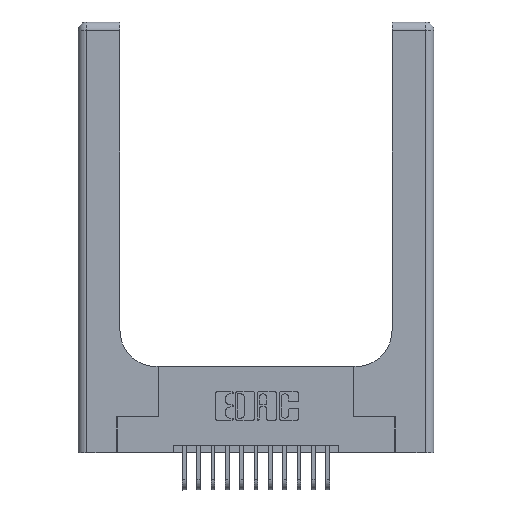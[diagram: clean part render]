
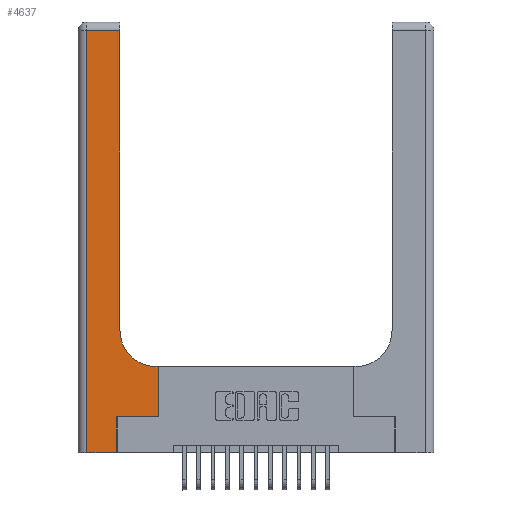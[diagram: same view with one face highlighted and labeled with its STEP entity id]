
A CAD part, top view. The second image highlights one B-rep face of the part: STEP entity #4637.
In plain terms, the highlighted planar face has unit normal (0, 0, 1).
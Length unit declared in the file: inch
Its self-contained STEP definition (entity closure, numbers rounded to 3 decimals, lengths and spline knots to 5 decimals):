
#248 = EDGE_CURVE ( 'NONE', #2853, #952, #790, .T. ) ;
#262 = LINE ( 'NONE', #1208, #7528 ) ;
#790 = LINE ( 'NONE', #9815, #4466 ) ;
#952 = VERTEX_POINT ( 'NONE', #16871 ) ;
#1208 = CARTESIAN_POINT ( 'NONE',  ( 0.269, 0.25, 0.37 ) ) ;
#1217 = ORIENTED_EDGE ( 'NONE', *, *, #9031, .T. ) ;
#1301 = CARTESIAN_POINT ( 'NONE',  ( 0.2915, 2.94, 0.37 ) ) ;
#1729 = ORIENTED_EDGE ( 'NONE', *, *, #12691, .T. ) ;
#1808 = VECTOR ( 'NONE', #4950, 39.37008 ) ;
#2254 = EDGE_CURVE ( 'NONE', #8453, #15381, #5851, .T. ) ;
#2398 = DIRECTION ( 'NONE',  ( 0., 1., 0. ) ) ;
#2740 = CARTESIAN_POINT ( 'NONE',  ( 0.5585, 0.6, 0.37 ) ) ;
#2793 = DIRECTION ( 'NONE',  ( -1., 0., 0. ) ) ;
#2853 = VERTEX_POINT ( 'NONE', #17217 ) ;
#3018 = DIRECTION ( 'NONE',  ( 0., 1., 0. ) ) ;
#3750 = VERTEX_POINT ( 'NONE', #16655 ) ;
#4372 = PLANE ( 'NONE',  #6452 ) ;
#4466 = VECTOR ( 'NONE', #14268, 39.37008 ) ;
#4471 = CARTESIAN_POINT ( 'NONE',  ( 0.2915, 3., 0.37 ) ) ;
#4545 = CARTESIAN_POINT ( 'NONE',  ( 0.5585, 0.25, 0.37 ) ) ;
#4637 = ADVANCED_FACE ( 'NONE', ( #17315 ), #4372, .F. ) ;
#4950 = DIRECTION ( 'NONE',  ( -1., 0., 0. ) ) ;
#4987 = EDGE_CURVE ( 'NONE', #15241, #11306, #12165, .T. ) ;
#4993 = VECTOR ( 'NONE', #3018, 39.37008 ) ;
#5088 = EDGE_CURVE ( 'NONE', #9762, #8453, #14529, .T. ) ;
#5576 = DIRECTION ( 'NONE',  ( 0., 0., -1. ) ) ;
#5727 = DIRECTION ( 'NONE',  ( -1., 0., 0. ) ) ;
#5851 = LINE ( 'NONE', #15827, #1808 ) ;
#6071 = DIRECTION ( 'NONE',  ( 0., -1., 0. ) ) ;
#6157 = LINE ( 'NONE', #14285, #17087 ) ;
#6452 = AXIS2_PLACEMENT_3D ( 'NONE', #8402, #13926, #5727 ) ;
#7070 = CARTESIAN_POINT ( 'NONE',  ( 0.06, 2.94, 0.37 ) ) ;
#7467 = VECTOR ( 'NONE', #2398, 39.37008 ) ;
#7528 = VECTOR ( 'NONE', #8007, 39.37008 ) ;
#8007 = DIRECTION ( 'NONE',  ( 1., 0., 0. ) ) ;
#8081 = VECTOR ( 'NONE', #14018, 39.37008 ) ;
#8162 = LINE ( 'NONE', #11180, #4993 ) ;
#8402 = CARTESIAN_POINT ( 'NONE',  ( 0., 3., 0.37 ) ) ;
#8453 = VERTEX_POINT ( 'NONE', #1301 ) ;
#8523 = VECTOR ( 'NONE', #2793, 39.37008 ) ;
#9031 = EDGE_CURVE ( 'NONE', #3750, #15424, #262, .T. ) ;
#9245 = EDGE_CURVE ( 'NONE', #15424, #15241, #8162, .T. ) ;
#9762 = VERTEX_POINT ( 'NONE', #12242 ) ;
#9815 = CARTESIAN_POINT ( 'NONE',  ( 0., 0., 0.37 ) ) ;
#10178 = EDGE_LOOP ( 'NONE', ( #13649, #10847, #17282, #11571, #13749, #1217, #10959, #10189, #1729 ) ) ;
#10189 = ORIENTED_EDGE ( 'NONE', *, *, #4987, .T. ) ;
#10813 = CARTESIAN_POINT ( 'NONE',  ( 0.5415, 0.6, 0.37 ) ) ;
#10847 = ORIENTED_EDGE ( 'NONE', *, *, #2254, .T. ) ;
#10958 = CARTESIAN_POINT ( 'NONE',  ( 0.2915, 0.6, 0.37 ) ) ;
#10959 = ORIENTED_EDGE ( 'NONE', *, *, #9245, .T. ) ;
#11180 = CARTESIAN_POINT ( 'NONE',  ( 0.5585, 0.25, 0.37 ) ) ;
#11306 = VERTEX_POINT ( 'NONE', #10813 ) ;
#11567 = CIRCLE ( 'NONE', #12018, 0.25 ) ;
#11571 = ORIENTED_EDGE ( 'NONE', *, *, #248, .T. ) ;
#12018 = AXIS2_PLACEMENT_3D ( 'NONE', #13751, #5576, #15139 ) ;
#12165 = LINE ( 'NONE', #10958, #8523 ) ;
#12242 = CARTESIAN_POINT ( 'NONE',  ( 0.2915, 0.85, 0.37 ) ) ;
#12691 = EDGE_CURVE ( 'NONE', #11306, #9762, #11567, .T. ) ;
#13162 = EDGE_CURVE ( 'NONE', #952, #3750, #14779, .T. ) ;
#13649 = ORIENTED_EDGE ( 'NONE', *, *, #5088, .T. ) ;
#13749 = ORIENTED_EDGE ( 'NONE', *, *, #13162, .T. ) ;
#13751 = CARTESIAN_POINT ( 'NONE',  ( 0.5415, 0.85, 0.37 ) ) ;
#13926 = DIRECTION ( 'NONE',  ( 0., 0., -1. ) ) ;
#14018 = DIRECTION ( 'NONE',  ( 0., 1., 0. ) ) ;
#14268 = DIRECTION ( 'NONE',  ( 1., 0., 0. ) ) ;
#14285 = CARTESIAN_POINT ( 'NONE',  ( 0.06, 3., 0.37 ) ) ;
#14529 = LINE ( 'NONE', #4471, #8081 ) ;
#14653 = CARTESIAN_POINT ( 'NONE',  ( 0.269, 0., 0.37 ) ) ;
#14779 = LINE ( 'NONE', #14653, #7467 ) ;
#14994 = EDGE_CURVE ( 'NONE', #15381, #2853, #6157, .T. ) ;
#15139 = DIRECTION ( 'NONE',  ( 1., 0., 0. ) ) ;
#15241 = VERTEX_POINT ( 'NONE', #2740 ) ;
#15381 = VERTEX_POINT ( 'NONE', #7070 ) ;
#15424 = VERTEX_POINT ( 'NONE', #4545 ) ;
#15827 = CARTESIAN_POINT ( 'NONE',  ( 0., 2.94, 0.37 ) ) ;
#16655 = CARTESIAN_POINT ( 'NONE',  ( 0.269, 0.25, 0.37 ) ) ;
#16871 = CARTESIAN_POINT ( 'NONE',  ( 0.269, 0., 0.37 ) ) ;
#17087 = VECTOR ( 'NONE', #6071, 39.37008 ) ;
#17217 = CARTESIAN_POINT ( 'NONE',  ( 0.06, 0., 0.37 ) ) ;
#17282 = ORIENTED_EDGE ( 'NONE', *, *, #14994, .T. ) ;
#17315 = FACE_OUTER_BOUND ( 'NONE', #10178, .T. ) ;
